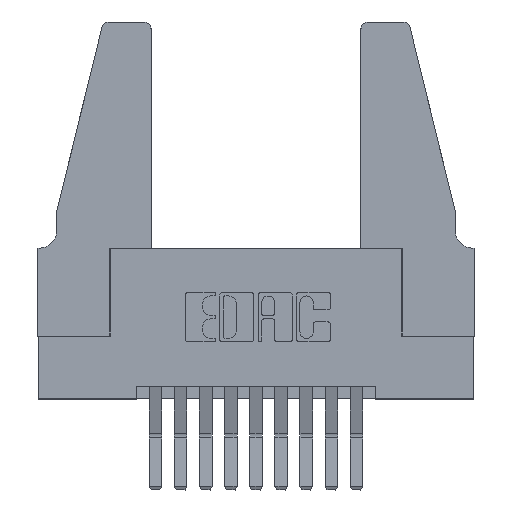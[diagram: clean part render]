
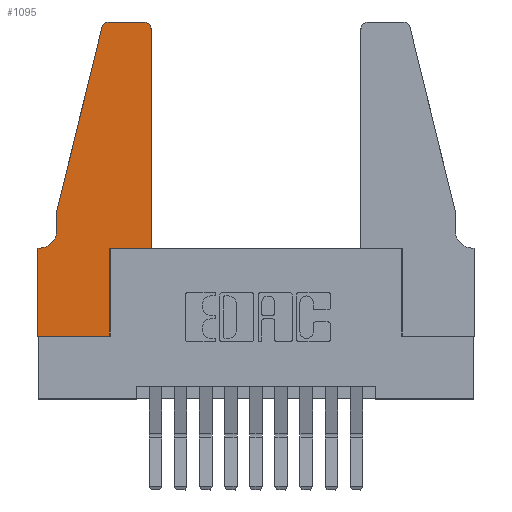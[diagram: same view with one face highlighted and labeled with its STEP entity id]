
A CAD part, top view. The second image highlights one B-rep face of the part: STEP entity #1095.
In plain terms, the highlighted planar face has unit normal (0, 0, 1).
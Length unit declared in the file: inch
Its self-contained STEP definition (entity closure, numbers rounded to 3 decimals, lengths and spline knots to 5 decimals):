
#172 = LINE ( 'NONE', #1839, #12960 ) ;
#193 = ORIENTED_EDGE ( 'NONE', *, *, #13241, .T. ) ;
#375 = DIRECTION ( 'NONE',  ( 0., 0., 1. ) ) ;
#550 = DIRECTION ( 'NONE',  ( 1., 0., 0. ) ) ;
#637 = ORIENTED_EDGE ( 'NONE', *, *, #11048, .T. ) ;
#748 = LINE ( 'NONE', #5305, #6394 ) ;
#786 = CARTESIAN_POINT ( 'NONE',  ( 0.0755, 0.5, 0.37 ) ) ;
#1037 = VECTOR ( 'NONE', #1151, 39.37008 ) ;
#1095 = ADVANCED_FACE ( 'NONE', ( #2017 ), #2461, .T. ) ;
#1151 = DIRECTION ( 'NONE',  ( 0., 1., 0. ) ) ;
#1164 = DIRECTION ( 'NONE',  ( 0., -1., 0. ) ) ;
#1329 = EDGE_CURVE ( 'NONE', #4488, #7465, #4990, .T. ) ;
#1634 = ORIENTED_EDGE ( 'NONE', *, *, #7481, .T. ) ;
#1798 = CARTESIAN_POINT ( 'NONE',  ( 0.4505, 0.35, 0.37 ) ) ;
#1839 = CARTESIAN_POINT ( 'NONE',  ( 0., 0., 0.37 ) ) ;
#2017 = FACE_OUTER_BOUND ( 'NONE', #9004, .T. ) ;
#2461 = PLANE ( 'NONE',  #11877 ) ;
#2471 = DIRECTION ( 'NONE',  ( 0., 0., 1. ) ) ;
#2517 = DIRECTION ( 'NONE',  ( 1., 0., 0. ) ) ;
#2595 = CARTESIAN_POINT ( 'NONE',  ( 0., 0.35, 0.37 ) ) ;
#2713 = CARTESIAN_POINT ( 'NONE',  ( 0.2865, 0.35, 0.37 ) ) ;
#2916 = DIRECTION ( 'NONE',  ( 0., -1., 0. ) ) ;
#2966 = DIRECTION ( 'NONE',  ( 0., 1., 0. ) ) ;
#3065 = VERTEX_POINT ( 'NONE', #10780 ) ;
#3252 = VERTEX_POINT ( 'NONE', #2713 ) ;
#3623 = ORIENTED_EDGE ( 'NONE', *, *, #1329, .T. ) ;
#3646 = EDGE_CURVE ( 'NONE', #6580, #11058, #12991, .T. ) ;
#3910 = ORIENTED_EDGE ( 'NONE', *, *, #8572, .T. ) ;
#3920 = AXIS2_PLACEMENT_3D ( 'NONE', #12481, #6122, #13565 ) ;
#4488 = VERTEX_POINT ( 'NONE', #7963 ) ;
#4614 = EDGE_CURVE ( 'NONE', #3252, #6580, #9120, .T. ) ;
#4680 = LINE ( 'NONE', #8575, #12787 ) ;
#4807 = CARTESIAN_POINT ( 'NONE',  ( 0.4505, 1.22, 0.37 ) ) ;
#4848 = EDGE_CURVE ( 'NONE', #9183, #6304, #5789, .T. ) ;
#4990 = LINE ( 'NONE', #786, #13115 ) ;
#5000 = DIRECTION ( 'NONE',  ( 1., 0., 0. ) ) ;
#5111 = VECTOR ( 'NONE', #6046, 39.37008 ) ;
#5151 = ORIENTED_EDGE ( 'NONE', *, *, #13198, .T. ) ;
#5305 = CARTESIAN_POINT ( 'NONE',  ( 0., 0., 0.37 ) ) ;
#5371 = CARTESIAN_POINT ( 'NONE',  ( 0.284, 1.25, 0.37 ) ) ;
#5695 = CIRCLE ( 'NONE', #7880, 0.03 ) ;
#5789 = LINE ( 'NONE', #8491, #8309 ) ;
#5824 = EDGE_CURVE ( 'NONE', #11058, #9183, #12237, .T. ) ;
#5840 = ORIENTED_EDGE ( 'NONE', *, *, #6627, .T. ) ;
#5904 = VERTEX_POINT ( 'NONE', #13193 ) ;
#6046 = DIRECTION ( 'NONE',  ( -1., 0., 0. ) ) ;
#6122 = DIRECTION ( 'NONE',  ( 0., 0., -1. ) ) ;
#6240 = AXIS2_PLACEMENT_3D ( 'NONE', #6729, #375, #7806 ) ;
#6304 = VERTEX_POINT ( 'NONE', #5371 ) ;
#6313 = CARTESIAN_POINT ( 'NONE',  ( 0.0755, 0.5, 0.37 ) ) ;
#6316 = ORIENTED_EDGE ( 'NONE', *, *, #4848, .T. ) ;
#6394 = VECTOR ( 'NONE', #8492, 39.37008 ) ;
#6580 = VERTEX_POINT ( 'NONE', #10217 ) ;
#6627 = EDGE_CURVE ( 'NONE', #5904, #12277, #13568, .T. ) ;
#6631 = DIRECTION ( 'NONE',  ( -0.239, -0.971, 0. ) ) ;
#6729 = CARTESIAN_POINT ( 'NONE',  ( 0.4205, 1.22, 0.37 ) ) ;
#6920 = DIRECTION ( 'NONE',  ( 0., 0., 1. ) ) ;
#7306 = CIRCLE ( 'NONE', #3920, 0.07 ) ;
#7465 = VERTEX_POINT ( 'NONE', #6313 ) ;
#7481 = EDGE_CURVE ( 'NONE', #12098, #11950, #748, .T. ) ;
#7806 = DIRECTION ( 'NONE',  ( 1., 0., 0. ) ) ;
#7880 = AXIS2_PLACEMENT_3D ( 'NONE', #13292, #6920, #550 ) ;
#7963 = CARTESIAN_POINT ( 'NONE',  ( 0.25487, 1.22718, 0.37 ) ) ;
#7974 = ORIENTED_EDGE ( 'NONE', *, *, #5824, .T. ) ;
#8309 = VECTOR ( 'NONE', #9554, 39.37008 ) ;
#8491 = CARTESIAN_POINT ( 'NONE',  ( 0.2605, 1.25, 0.37 ) ) ;
#8492 = DIRECTION ( 'NONE',  ( 1., 0., 0. ) ) ;
#8564 = CARTESIAN_POINT ( 'NONE',  ( 0.4505, 0.35, 0.37 ) ) ;
#8572 = EDGE_CURVE ( 'NONE', #11950, #3252, #11910, .T. ) ;
#8575 = CARTESIAN_POINT ( 'NONE',  ( 0.0755, 0.5, 0.37 ) ) ;
#9004 = EDGE_LOOP ( 'NONE', ( #6316, #637, #3623, #10164, #193, #5840, #5151, #1634, #3910, #10033, #13649, #7974 ) ) ;
#9120 = LINE ( 'NONE', #1798, #10928 ) ;
#9183 = VERTEX_POINT ( 'NONE', #11235 ) ;
#9554 = DIRECTION ( 'NONE',  ( -1., 0., 0. ) ) ;
#10033 = ORIENTED_EDGE ( 'NONE', *, *, #4614, .T. ) ;
#10164 = ORIENTED_EDGE ( 'NONE', *, *, #13433, .T. ) ;
#10217 = CARTESIAN_POINT ( 'NONE',  ( 0.4505, 0.35, 0.37 ) ) ;
#10265 = CARTESIAN_POINT ( 'NONE',  ( 0.2865, 0., 0.37 ) ) ;
#10780 = CARTESIAN_POINT ( 'NONE',  ( 0.0755, 0.42, 0.37 ) ) ;
#10928 = VECTOR ( 'NONE', #5000, 39.37008 ) ;
#11048 = EDGE_CURVE ( 'NONE', #6304, #4488, #5695, .T. ) ;
#11058 = VERTEX_POINT ( 'NONE', #4807 ) ;
#11235 = CARTESIAN_POINT ( 'NONE',  ( 0.4205, 1.25, 0.37 ) ) ;
#11308 = CARTESIAN_POINT ( 'NONE',  ( 0.0755, 0.35, 0.37 ) ) ;
#11835 = CARTESIAN_POINT ( 'NONE',  ( 0., 0.35, 0.37 ) ) ;
#11877 = AXIS2_PLACEMENT_3D ( 'NONE', #2595, #2471, #2517 ) ;
#11910 = LINE ( 'NONE', #13533, #12248 ) ;
#11950 = VERTEX_POINT ( 'NONE', #10265 ) ;
#12098 = VERTEX_POINT ( 'NONE', #13683 ) ;
#12237 = CIRCLE ( 'NONE', #6240, 0.03 ) ;
#12248 = VECTOR ( 'NONE', #2966, 39.37008 ) ;
#12277 = VERTEX_POINT ( 'NONE', #11835 ) ;
#12481 = CARTESIAN_POINT ( 'NONE',  ( 0.0055, 0.42, 0.37 ) ) ;
#12787 = VECTOR ( 'NONE', #1164, 39.37008 ) ;
#12960 = VECTOR ( 'NONE', #2916, 39.37008 ) ;
#12991 = LINE ( 'NONE', #8564, #1037 ) ;
#13115 = VECTOR ( 'NONE', #6631, 39.37008 ) ;
#13193 = CARTESIAN_POINT ( 'NONE',  ( 0.0055, 0.35, 0.37 ) ) ;
#13198 = EDGE_CURVE ( 'NONE', #12277, #12098, #172, .T. ) ;
#13241 = EDGE_CURVE ( 'NONE', #3065, #5904, #7306, .T. ) ;
#13292 = CARTESIAN_POINT ( 'NONE',  ( 0.284, 1.22, 0.37 ) ) ;
#13433 = EDGE_CURVE ( 'NONE', #7465, #3065, #4680, .T. ) ;
#13533 = CARTESIAN_POINT ( 'NONE',  ( 0.2865, 0.35, 0.37 ) ) ;
#13565 = DIRECTION ( 'NONE',  ( -1., 0., 0. ) ) ;
#13568 = LINE ( 'NONE', #11308, #5111 ) ;
#13649 = ORIENTED_EDGE ( 'NONE', *, *, #3646, .T. ) ;
#13683 = CARTESIAN_POINT ( 'NONE',  ( 0., 0., 0.37 ) ) ;
